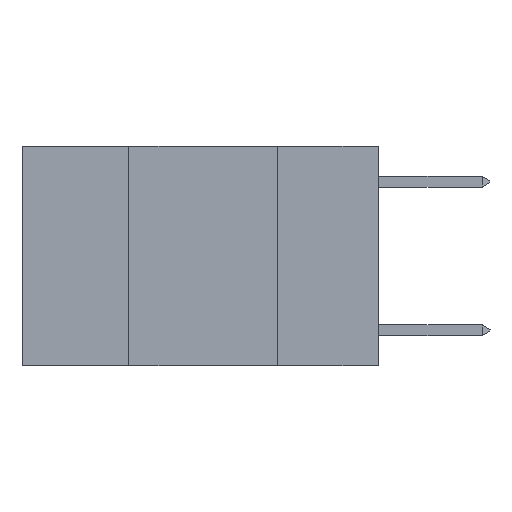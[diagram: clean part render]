
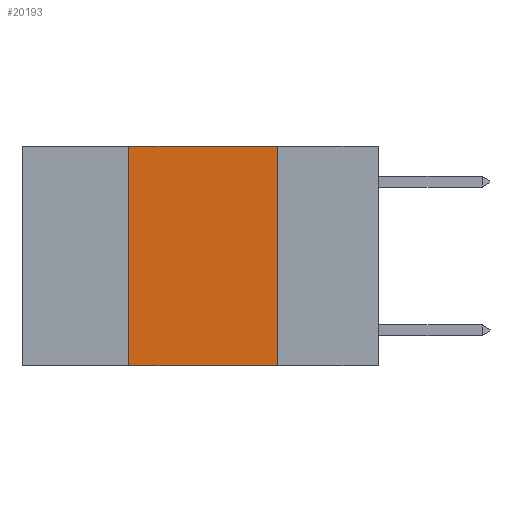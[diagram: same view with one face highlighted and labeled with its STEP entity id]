
A CAD part, left-side view. The second image highlights one B-rep face of the part: STEP entity #20193.
In plain terms, the highlighted planar face has unit normal (-1, 0, 0).
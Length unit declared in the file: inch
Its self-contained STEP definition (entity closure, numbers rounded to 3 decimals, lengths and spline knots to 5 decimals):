
#631 = AXIS2_PLACEMENT_3D ( 'NONE', #2240, #4833, #22536 ) ;
#2240 = CARTESIAN_POINT ( 'NONE',  ( 0., 0.6, 0. ) ) ;
#2706 = LINE ( 'NONE', #5584, #14612 ) ;
#3970 = CARTESIAN_POINT ( 'NONE',  ( 0., 0.17, 0. ) ) ;
#4833 = DIRECTION ( 'NONE',  ( 1., 0., 0. ) ) ;
#5053 = VECTOR ( 'NONE', #6494, 39.37008 ) ;
#5122 = VECTOR ( 'NONE', #25609, 39.37008 ) ;
#5584 = CARTESIAN_POINT ( 'NONE',  ( 0., 0.42, 0. ) ) ;
#6020 = ORIENTED_EDGE ( 'NONE', *, *, #30357, .F. ) ;
#6494 = DIRECTION ( 'NONE',  ( 0., 0., -1. ) ) ;
#6987 = LINE ( 'NONE', #10755, #7798 ) ;
#7798 = VECTOR ( 'NONE', #15827, 39.37008 ) ;
#8151 = DIRECTION ( 'NONE',  ( 0., 0., 1. ) ) ;
#8174 = VERTEX_POINT ( 'NONE', #11811 ) ;
#8980 = CARTESIAN_POINT ( 'NONE',  ( 0., 0.42, -0.37 ) ) ;
#10594 = CARTESIAN_POINT ( 'NONE',  ( 0., 0.6, -0.37 ) ) ;
#10755 = CARTESIAN_POINT ( 'NONE',  ( 0., 0.6, 0. ) ) ;
#11791 = LINE ( 'NONE', #3970, #5053 ) ;
#11811 = CARTESIAN_POINT ( 'NONE',  ( 0., 0.42, 0. ) ) ;
#11858 = LINE ( 'NONE', #10594, #5122 ) ;
#14612 = VECTOR ( 'NONE', #8151, 39.37008 ) ;
#15080 = EDGE_CURVE ( 'NONE', #32005, #26576, #11858, .T. ) ;
#15827 = DIRECTION ( 'NONE',  ( 0., -1., 0. ) ) ;
#15990 = EDGE_CURVE ( 'NONE', #24714, #26576, #11791, .T. ) ;
#16920 = ORIENTED_EDGE ( 'NONE', *, *, #24907, .F. ) ;
#17490 = PLANE ( 'NONE',  #631 ) ;
#18414 = FACE_OUTER_BOUND ( 'NONE', #21003, .T. ) ;
#20193 = ADVANCED_FACE ( 'NONE', ( #18414 ), #17490, .F. ) ;
#21003 = EDGE_LOOP ( 'NONE', ( #30142, #16920, #6020, #29613 ) ) ;
#22536 = DIRECTION ( 'NONE',  ( 0., 0., -1. ) ) ;
#24714 = VERTEX_POINT ( 'NONE', #27523 ) ;
#24907 = EDGE_CURVE ( 'NONE', #8174, #24714, #6987, .T. ) ;
#25609 = DIRECTION ( 'NONE',  ( 0., -1., 0. ) ) ;
#26576 = VERTEX_POINT ( 'NONE', #31822 ) ;
#27523 = CARTESIAN_POINT ( 'NONE',  ( 0., 0.17, 0. ) ) ;
#29613 = ORIENTED_EDGE ( 'NONE', *, *, #15080, .T. ) ;
#30142 = ORIENTED_EDGE ( 'NONE', *, *, #15990, .F. ) ;
#30357 = EDGE_CURVE ( 'NONE', #32005, #8174, #2706, .T. ) ;
#31822 = CARTESIAN_POINT ( 'NONE',  ( 0., 0.17, -0.37 ) ) ;
#32005 = VERTEX_POINT ( 'NONE', #8980 ) ;
